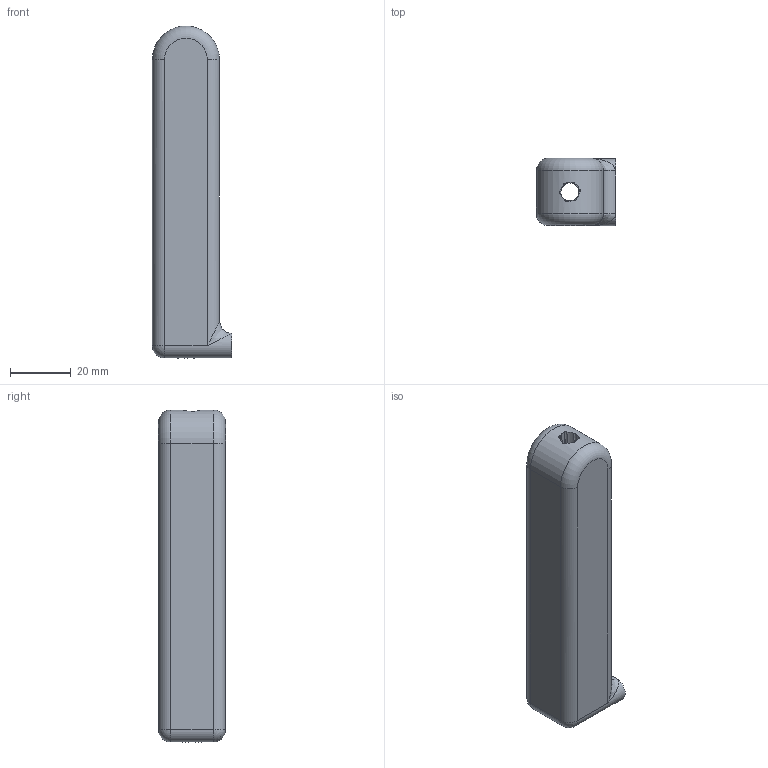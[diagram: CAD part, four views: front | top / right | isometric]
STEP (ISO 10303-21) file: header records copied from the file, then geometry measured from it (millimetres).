
FILE_DESCRIPTION((''),'2;1');
FILE_NAME('PM422Barrel2v2.stp','2015-08-22T19:05:11',('JamesRPatrick'),(''),'Autodesk Inventor 2012','Autodesk Inventor 2012','');
FILE_SCHEMA(('AUTOMOTIVE_DESIGN { 1 0 10303 214 1 1 1 1 }'));
Length unit declared in the file: millimetre
Products named in the file (1): PM422Barrel2v2
Bounding box: 26 x 22 x 109 mm (x, y, z)
Volume: 47212.4 mm3; surface area: 11738.1 mm2
Topology: 1 solids, 1 shells, 48 faces, 117 edges, 68 vertices
Faces by surface type: bspline 17, cylinder 15, plane 12, sphere 2, torus 2
Entity records: 2330 total; most frequent: CARTESIAN_POINT 1354, ORIENTED_EDGE 224, DIRECTION 151, EDGE_CURVE 112, AXIS2_PLACEMENT_3D 66, VERTEX_POINT 66, B_SPLINE_CURVE_WITH_KNOTS 59, EDGE_LOOP 50
